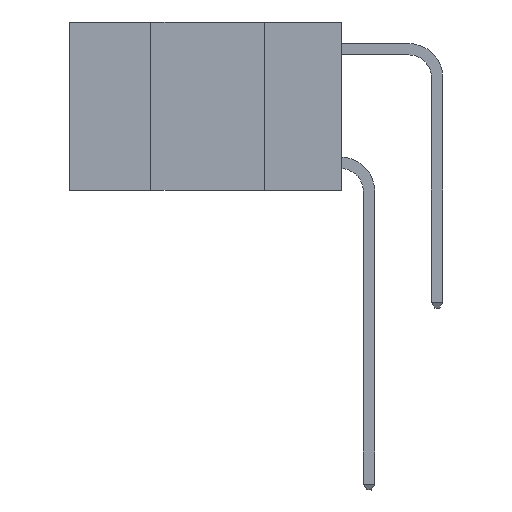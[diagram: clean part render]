
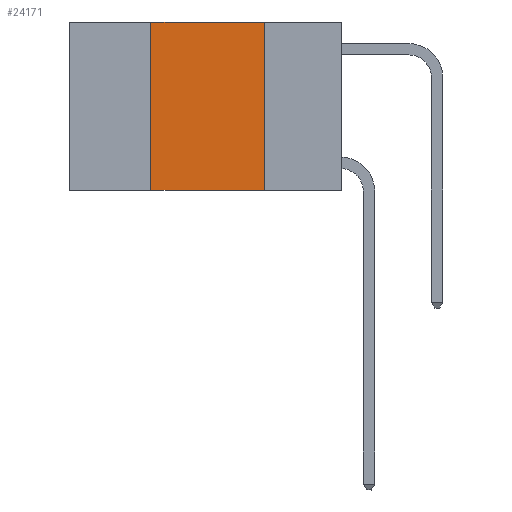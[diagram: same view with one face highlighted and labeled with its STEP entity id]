
A CAD part, left-side view. The second image highlights one B-rep face of the part: STEP entity #24171.
In plain terms, the highlighted planar face has unit normal (-1, 0, 0).
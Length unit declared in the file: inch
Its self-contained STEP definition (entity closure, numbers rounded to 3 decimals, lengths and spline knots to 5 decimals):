
#463 = ORIENTED_EDGE ( 'NONE', *, *, #31362, .F. ) ;
#2510 = AXIS2_PLACEMENT_3D ( 'NONE', #14631, #31824, #17091 ) ;
#3844 = CARTESIAN_POINT ( 'NONE',  ( 0., 0.6, -0.37 ) ) ;
#4790 = VERTEX_POINT ( 'NONE', #13761 ) ;
#8711 = ORIENTED_EDGE ( 'NONE', *, *, #28802, .F. ) ;
#9495 = CARTESIAN_POINT ( 'NONE',  ( 0., 0.42, -0.37 ) ) ;
#9728 = DIRECTION ( 'NONE',  ( 0., 0., -1. ) ) ;
#12147 = PLANE ( 'NONE',  #2510 ) ;
#13453 = EDGE_LOOP ( 'NONE', ( #8711, #21286, #463, #17664 ) ) ;
#13761 = CARTESIAN_POINT ( 'NONE',  ( 0., 0.42, 0. ) ) ;
#13777 = DIRECTION ( 'NONE',  ( 0., 0., 1. ) ) ;
#13794 = DIRECTION ( 'NONE',  ( 0., -1., 0. ) ) ;
#14202 = CARTESIAN_POINT ( 'NONE',  ( 0., 0.17, -0.37 ) ) ;
#14631 = CARTESIAN_POINT ( 'NONE',  ( 0., 0.6, 0. ) ) ;
#15456 = EDGE_CURVE ( 'NONE', #28790, #28030, #31435, .T. ) ;
#17091 = DIRECTION ( 'NONE',  ( 0., 0., -1. ) ) ;
#17664 = ORIENTED_EDGE ( 'NONE', *, *, #15456, .T. ) ;
#18013 = LINE ( 'NONE', #26958, #31103 ) ;
#19056 = FACE_OUTER_BOUND ( 'NONE', #13453, .T. ) ;
#19506 = DIRECTION ( 'NONE',  ( 0., -1., 0. ) ) ;
#20634 = LINE ( 'NONE', #26066, #26416 ) ;
#20684 = VERTEX_POINT ( 'NONE', #28958 ) ;
#21286 = ORIENTED_EDGE ( 'NONE', *, *, #29426, .F. ) ;
#21916 = VECTOR ( 'NONE', #9728, 39.37008 ) ;
#24171 = ADVANCED_FACE ( 'NONE', ( #19056 ), #12147, .F. ) ;
#24505 = CARTESIAN_POINT ( 'NONE',  ( 0., 0.17, 0. ) ) ;
#24914 = VECTOR ( 'NONE', #13794, 39.37008 ) ;
#26066 = CARTESIAN_POINT ( 'NONE',  ( 0., 0.42, 0. ) ) ;
#26416 = VECTOR ( 'NONE', #13777, 39.37008 ) ;
#26958 = CARTESIAN_POINT ( 'NONE',  ( 0., 0.6, 0. ) ) ;
#28030 = VERTEX_POINT ( 'NONE', #14202 ) ;
#28465 = LINE ( 'NONE', #24505, #21916 ) ;
#28790 = VERTEX_POINT ( 'NONE', #9495 ) ;
#28802 = EDGE_CURVE ( 'NONE', #20684, #28030, #28465, .T. ) ;
#28958 = CARTESIAN_POINT ( 'NONE',  ( 0., 0.17, 0. ) ) ;
#29426 = EDGE_CURVE ( 'NONE', #4790, #20684, #18013, .T. ) ;
#31103 = VECTOR ( 'NONE', #19506, 39.37008 ) ;
#31362 = EDGE_CURVE ( 'NONE', #28790, #4790, #20634, .T. ) ;
#31435 = LINE ( 'NONE', #3844, #24914 ) ;
#31824 = DIRECTION ( 'NONE',  ( 1., 0., 0. ) ) ;
